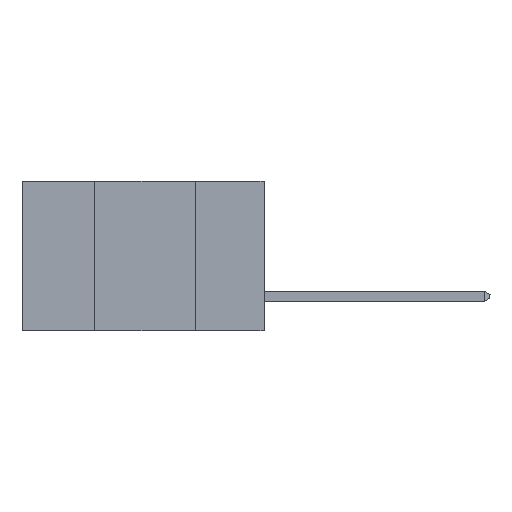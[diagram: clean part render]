
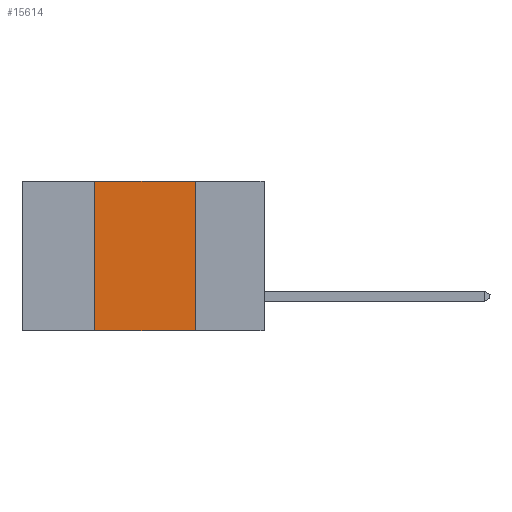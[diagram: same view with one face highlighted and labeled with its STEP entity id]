
A CAD part, left-side view. The second image highlights one B-rep face of the part: STEP entity #15614.
In plain terms, the highlighted planar face has unit normal (-1, 0, 0).
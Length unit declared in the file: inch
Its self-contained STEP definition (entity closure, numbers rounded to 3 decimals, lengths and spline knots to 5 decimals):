
#148 = EDGE_CURVE ( 'NONE', #7190, #15864, #3289, .T. ) ;
#238 = LINE ( 'NONE', #15062, #10929 ) ;
#577 = LINE ( 'NONE', #14895, #13000 ) ;
#674 = EDGE_CURVE ( 'NONE', #8760, #13886, #14238, .T. ) ;
#1126 = DIRECTION ( 'NONE',  ( 0., 0., 1. ) ) ;
#1481 = ORIENTED_EDGE ( 'NONE', *, *, #148, .F. ) ;
#2006 = DIRECTION ( 'NONE',  ( 1., 0., 0. ) ) ;
#2367 = CARTESIAN_POINT ( 'NONE',  ( 0., 0.42, 0. ) ) ;
#2841 = VECTOR ( 'NONE', #13367, 39.37008 ) ;
#3289 = LINE ( 'NONE', #2367, #9070 ) ;
#3631 = CARTESIAN_POINT ( 'NONE',  ( 0., 0.42, -0.37 ) ) ;
#3760 = CARTESIAN_POINT ( 'NONE',  ( 0., 0.17, -0.37 ) ) ;
#4212 = CARTESIAN_POINT ( 'NONE',  ( 0., 0.17, 0. ) ) ;
#4273 = EDGE_CURVE ( 'NONE', #15864, #8760, #238, .T. ) ;
#5004 = DIRECTION ( 'NONE',  ( 0., -1., 0. ) ) ;
#5913 = CARTESIAN_POINT ( 'NONE',  ( 0., 0.42, 0. ) ) ;
#5916 = ORIENTED_EDGE ( 'NONE', *, *, #4273, .F. ) ;
#6058 = CARTESIAN_POINT ( 'NONE',  ( 0., 0.6, 0. ) ) ;
#6846 = DIRECTION ( 'NONE',  ( 0., -1., 0. ) ) ;
#7190 = VERTEX_POINT ( 'NONE', #3631 ) ;
#8760 = VERTEX_POINT ( 'NONE', #11405 ) ;
#9070 = VECTOR ( 'NONE', #1126, 39.37008 ) ;
#9820 = FACE_OUTER_BOUND ( 'NONE', #14523, .T. ) ;
#10481 = AXIS2_PLACEMENT_3D ( 'NONE', #6058, #2006, #14318 ) ;
#10929 = VECTOR ( 'NONE', #6846, 39.37008 ) ;
#11185 = ORIENTED_EDGE ( 'NONE', *, *, #11439, .T. ) ;
#11405 = CARTESIAN_POINT ( 'NONE',  ( 0., 0.17, 0. ) ) ;
#11439 = EDGE_CURVE ( 'NONE', #7190, #13886, #577, .T. ) ;
#11722 = PLANE ( 'NONE',  #10481 ) ;
#11854 = ORIENTED_EDGE ( 'NONE', *, *, #674, .F. ) ;
#13000 = VECTOR ( 'NONE', #5004, 39.37008 ) ;
#13367 = DIRECTION ( 'NONE',  ( 0., 0., -1. ) ) ;
#13886 = VERTEX_POINT ( 'NONE', #3760 ) ;
#14238 = LINE ( 'NONE', #4212, #2841 ) ;
#14318 = DIRECTION ( 'NONE',  ( 0., 0., -1. ) ) ;
#14523 = EDGE_LOOP ( 'NONE', ( #11854, #5916, #1481, #11185 ) ) ;
#14895 = CARTESIAN_POINT ( 'NONE',  ( 0., 0.6, -0.37 ) ) ;
#15062 = CARTESIAN_POINT ( 'NONE',  ( 0., 0.6, 0. ) ) ;
#15614 = ADVANCED_FACE ( 'NONE', ( #9820 ), #11722, .F. ) ;
#15864 = VERTEX_POINT ( 'NONE', #5913 ) ;
